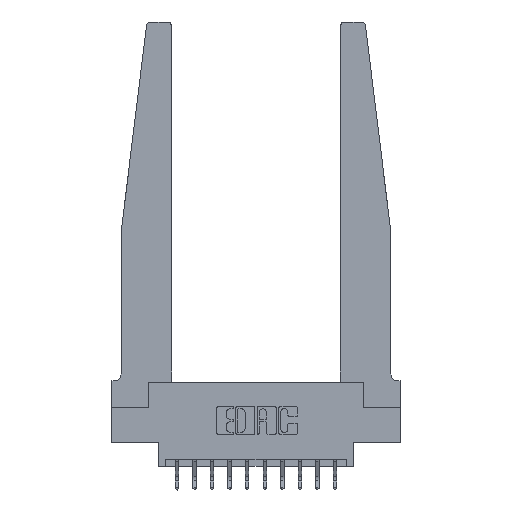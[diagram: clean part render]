
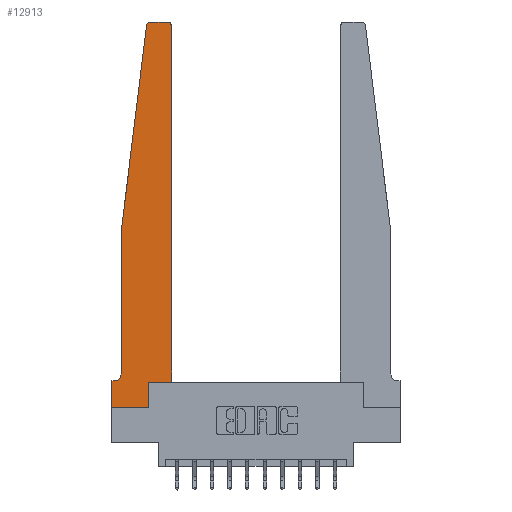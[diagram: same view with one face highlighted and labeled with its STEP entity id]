
A CAD part, top view. The second image highlights one B-rep face of the part: STEP entity #12913.
In plain terms, the highlighted planar face has unit normal (0, 0, 1).
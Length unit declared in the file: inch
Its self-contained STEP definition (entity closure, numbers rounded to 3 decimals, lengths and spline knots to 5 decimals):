
#8 = CARTESIAN_POINT ( 'NONE',  ( 0., 0.1875, 0.37 ) ) ;
#301 = VERTEX_POINT ( 'NONE', #15255 ) ;
#440 = VECTOR ( 'NONE', #2590, 39.37008 ) ;
#570 = CARTESIAN_POINT ( 'NONE',  ( 0.395, 2.75, 0.37 ) ) ;
#577 = EDGE_CURVE ( 'NONE', #7376, #7408, #8336, .T. ) ;
#666 = LINE ( 'NONE', #2438, #7182 ) ;
#705 = DIRECTION ( 'NONE',  ( 0., 1., 0. ) ) ;
#1042 = CARTESIAN_POINT ( 'NONE',  ( 0.015, 0.2375, 0.37 ) ) ;
#1145 = EDGE_CURVE ( 'NONE', #15050, #14408, #666, .T. ) ;
#1150 = VERTEX_POINT ( 'NONE', #13524 ) ;
#1152 = ORIENTED_EDGE ( 'NONE', *, *, #577, .T. ) ;
#1267 = DIRECTION ( 'NONE',  ( -1., 0., 0. ) ) ;
#1271 = EDGE_CURVE ( 'NONE', #14408, #13240, #8510, .T. ) ;
#1400 = EDGE_LOOP ( 'NONE', ( #3883, #6149, #2911, #15238, #5380, #11539, #1723, #11143, #14084, #4812, #10952, #1152 ) ) ;
#1723 = ORIENTED_EDGE ( 'NONE', *, *, #5608, .T. ) ;
#1936 = EDGE_CURVE ( 'NONE', #12337, #1150, #9852, .T. ) ;
#2271 = DIRECTION ( 'NONE',  ( -1., 0., 0. ) ) ;
#2438 = CARTESIAN_POINT ( 'NONE',  ( 0., 0., 0.37 ) ) ;
#2554 = DIRECTION ( 'NONE',  ( -1., 0., 0. ) ) ;
#2582 = CARTESIAN_POINT ( 'NONE',  ( 0.425, 0.18, 0.37 ) ) ;
#2590 = DIRECTION ( 'NONE',  ( 0., -1., 0. ) ) ;
#2825 = CARTESIAN_POINT ( 'NONE',  ( 0.065, 1.25, 0.37 ) ) ;
#2911 = ORIENTED_EDGE ( 'NONE', *, *, #15947, .T. ) ;
#2915 = CARTESIAN_POINT ( 'NONE',  ( 0., 0.1875, 0.37 ) ) ;
#3713 = CARTESIAN_POINT ( 'NONE',  ( 0.2605, 0.18, 0.37 ) ) ;
#3772 = CARTESIAN_POINT ( 'NONE',  ( 0.015, 0.1875, 0.37 ) ) ;
#3883 = ORIENTED_EDGE ( 'NONE', *, *, #13274, .T. ) ;
#3911 = CARTESIAN_POINT ( 'NONE',  ( 0.2605, 0.18, 0.37 ) ) ;
#3961 = DIRECTION ( 'NONE',  ( 0., 0., 1. ) ) ;
#3981 = VERTEX_POINT ( 'NONE', #2582 ) ;
#4127 = VECTOR ( 'NONE', #15881, 39.37008 ) ;
#4156 = DIRECTION ( 'NONE',  ( 0., 0., 1. ) ) ;
#4282 = DIRECTION ( 'NONE',  ( 1., 0., 0. ) ) ;
#4597 = VERTEX_POINT ( 'NONE', #8 ) ;
#4614 = EDGE_CURVE ( 'NONE', #13240, #3981, #13981, .T. ) ;
#4782 = CARTESIAN_POINT ( 'NONE',  ( 0., 0., 0.37 ) ) ;
#4812 = ORIENTED_EDGE ( 'NONE', *, *, #4614, .T. ) ;
#4992 = AXIS2_PLACEMENT_3D ( 'NONE', #5671, #3961, #4282 ) ;
#5380 = ORIENTED_EDGE ( 'NONE', *, *, #15016, .T. ) ;
#5391 = LINE ( 'NONE', #12978, #11551 ) ;
#5577 = AXIS2_PLACEMENT_3D ( 'NONE', #2915, #4156, #12738 ) ;
#5608 = EDGE_CURVE ( 'NONE', #4597, #15050, #7355, .T. ) ;
#5660 = CIRCLE ( 'NONE', #9481, 0.05 ) ;
#5664 = VECTOR ( 'NONE', #12483, 39.37008 ) ;
#5671 = CARTESIAN_POINT ( 'NONE',  ( 0.395, 2.72, 0.37 ) ) ;
#5997 = VECTOR ( 'NONE', #13906, 39.37008 ) ;
#6149 = ORIENTED_EDGE ( 'NONE', *, *, #11783, .T. ) ;
#6203 = CARTESIAN_POINT ( 'NONE',  ( 0.425, 0.18, 0.37 ) ) ;
#6863 = FACE_OUTER_BOUND ( 'NONE', #1400, .T. ) ;
#7087 = CARTESIAN_POINT ( 'NONE',  ( 0.27653, 2.72, 0.37 ) ) ;
#7182 = VECTOR ( 'NONE', #9781, 39.37008 ) ;
#7214 = CARTESIAN_POINT ( 'NONE',  ( 0., 0., 0.37 ) ) ;
#7355 = LINE ( 'NONE', #4782, #4127 ) ;
#7376 = VERTEX_POINT ( 'NONE', #14045 ) ;
#7408 = VERTEX_POINT ( 'NONE', #570 ) ;
#8049 = EDGE_CURVE ( 'NONE', #3981, #7376, #5391, .T. ) ;
#8309 = DIRECTION ( 'NONE',  ( 1., 0., 0. ) ) ;
#8336 = CIRCLE ( 'NONE', #4992, 0.03 ) ;
#8510 = LINE ( 'NONE', #3911, #5664 ) ;
#8750 = VECTOR ( 'NONE', #1267, 39.37008 ) ;
#9255 = LINE ( 'NONE', #2825, #5997 ) ;
#9481 = AXIS2_PLACEMENT_3D ( 'NONE', #1042, #9624, #2271 ) ;
#9577 = CIRCLE ( 'NONE', #12092, 0.03 ) ;
#9624 = DIRECTION ( 'NONE',  ( 0., 0., -1. ) ) ;
#9652 = CARTESIAN_POINT ( 'NONE',  ( 0.2605, 0., 0.37 ) ) ;
#9679 = EDGE_CURVE ( 'NONE', #14657, #4597, #11699, .T. ) ;
#9781 = DIRECTION ( 'NONE',  ( 1., 0., 0. ) ) ;
#9852 = LINE ( 'NONE', #14923, #440 ) ;
#10258 = PLANE ( 'NONE',  #5577 ) ;
#10952 = ORIENTED_EDGE ( 'NONE', *, *, #8049, .T. ) ;
#11052 = VERTEX_POINT ( 'NONE', #14116 ) ;
#11137 = CARTESIAN_POINT ( 'NONE',  ( 0.065, 0.1875, 0.37 ) ) ;
#11143 = ORIENTED_EDGE ( 'NONE', *, *, #1145, .T. ) ;
#11539 = ORIENTED_EDGE ( 'NONE', *, *, #9679, .T. ) ;
#11551 = VECTOR ( 'NONE', #705, 39.37008 ) ;
#11699 = LINE ( 'NONE', #11137, #14993 ) ;
#11783 = EDGE_CURVE ( 'NONE', #11052, #301, #9577, .T. ) ;
#12092 = AXIS2_PLACEMENT_3D ( 'NONE', #7087, #15726, #8309 ) ;
#12337 = VERTEX_POINT ( 'NONE', #14081 ) ;
#12483 = DIRECTION ( 'NONE',  ( 0., 1., 0. ) ) ;
#12738 = DIRECTION ( 'NONE',  ( 1., 0., 0. ) ) ;
#12913 = ADVANCED_FACE ( 'NONE', ( #6863 ), #10258, .T. ) ;
#12978 = CARTESIAN_POINT ( 'NONE',  ( 0.425, 0.18, 0.37 ) ) ;
#13240 = VERTEX_POINT ( 'NONE', #3713 ) ;
#13274 = EDGE_CURVE ( 'NONE', #7408, #11052, #14968, .T. ) ;
#13524 = CARTESIAN_POINT ( 'NONE',  ( 0.065, 0.2375, 0.37 ) ) ;
#13550 = CARTESIAN_POINT ( 'NONE',  ( 0.25, 2.75, 0.37 ) ) ;
#13906 = DIRECTION ( 'NONE',  ( -0.122, -0.992, 0. ) ) ;
#13981 = LINE ( 'NONE', #6203, #14373 ) ;
#14045 = CARTESIAN_POINT ( 'NONE',  ( 0.425, 2.72, 0.37 ) ) ;
#14081 = CARTESIAN_POINT ( 'NONE',  ( 0.065, 1.25, 0.37 ) ) ;
#14084 = ORIENTED_EDGE ( 'NONE', *, *, #1271, .T. ) ;
#14116 = CARTESIAN_POINT ( 'NONE',  ( 0.27653, 2.75, 0.37 ) ) ;
#14373 = VECTOR ( 'NONE', #14839, 39.37008 ) ;
#14408 = VERTEX_POINT ( 'NONE', #9652 ) ;
#14657 = VERTEX_POINT ( 'NONE', #3772 ) ;
#14839 = DIRECTION ( 'NONE',  ( 1., 0., 0. ) ) ;
#14923 = CARTESIAN_POINT ( 'NONE',  ( 0.065, 1.25, 0.37 ) ) ;
#14968 = LINE ( 'NONE', #13550, #8750 ) ;
#14993 = VECTOR ( 'NONE', #2554, 39.37008 ) ;
#15016 = EDGE_CURVE ( 'NONE', #1150, #14657, #5660, .T. ) ;
#15050 = VERTEX_POINT ( 'NONE', #7214 ) ;
#15238 = ORIENTED_EDGE ( 'NONE', *, *, #1936, .T. ) ;
#15255 = CARTESIAN_POINT ( 'NONE',  ( 0.24675, 2.72367, 0.37 ) ) ;
#15726 = DIRECTION ( 'NONE',  ( 0., 0., 1. ) ) ;
#15881 = DIRECTION ( 'NONE',  ( 0., -1., 0. ) ) ;
#15947 = EDGE_CURVE ( 'NONE', #301, #12337, #9255, .T. ) ;
